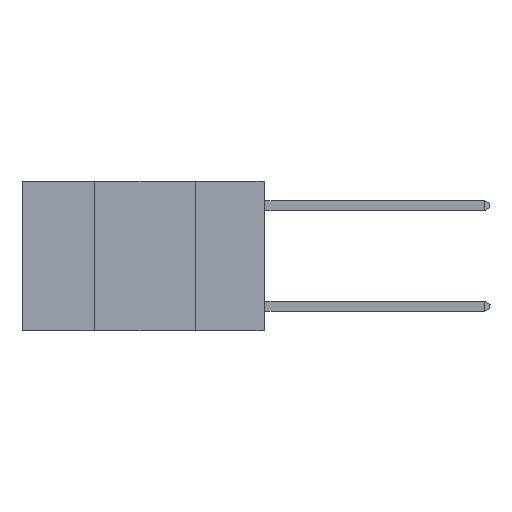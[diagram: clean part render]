
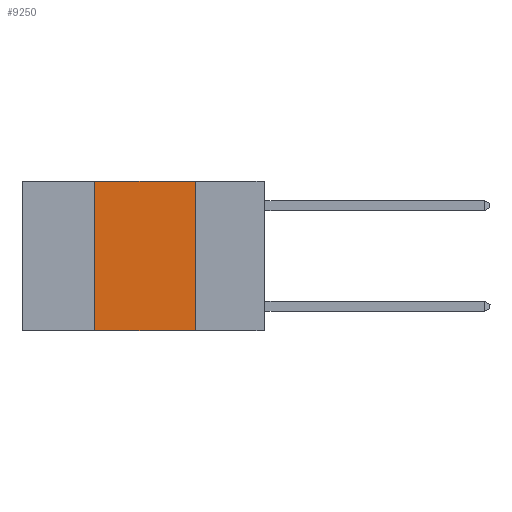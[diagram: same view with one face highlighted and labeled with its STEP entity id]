
A CAD part, left-side view. The second image highlights one B-rep face of the part: STEP entity #9250.
In plain terms, the highlighted planar face has unit normal (-1, 0, 0).
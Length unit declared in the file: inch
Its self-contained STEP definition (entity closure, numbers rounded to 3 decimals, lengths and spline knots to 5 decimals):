
#899 = VECTOR ( 'NONE', #6600, 39.37008 ) ;
#1778 = DIRECTION ( 'NONE',  ( 1., 0., 0. ) ) ;
#2074 = CARTESIAN_POINT ( 'NONE',  ( 0., 0.17, 0. ) ) ;
#2697 = DIRECTION ( 'NONE',  ( 0., -1., 0. ) ) ;
#2710 = VECTOR ( 'NONE', #13397, 39.37008 ) ;
#3205 = ORIENTED_EDGE ( 'NONE', *, *, #10799, .F. ) ;
#3374 = ORIENTED_EDGE ( 'NONE', *, *, #15927, .T. ) ;
#3683 = VERTEX_POINT ( 'NONE', #12729 ) ;
#3836 = LINE ( 'NONE', #6655, #899 ) ;
#3963 = EDGE_LOOP ( 'NONE', ( #3205, #9900, #13261, #3374 ) ) ;
#4249 = LINE ( 'NONE', #9937, #13894 ) ;
#5135 = CARTESIAN_POINT ( 'NONE',  ( 0., 0.17, -0.37 ) ) ;
#6184 = DIRECTION ( 'NONE',  ( 0., 0., 1. ) ) ;
#6420 = CARTESIAN_POINT ( 'NONE',  ( 0., 0.6, -0.37 ) ) ;
#6600 = DIRECTION ( 'NONE',  ( 0., -1., 0. ) ) ;
#6655 = CARTESIAN_POINT ( 'NONE',  ( 0., 0.6, 0. ) ) ;
#7323 = CARTESIAN_POINT ( 'NONE',  ( 0., 0.17, 0. ) ) ;
#8259 = EDGE_CURVE ( 'NONE', #11258, #3683, #4249, .T. ) ;
#8358 = VERTEX_POINT ( 'NONE', #5135 ) ;
#9023 = FACE_OUTER_BOUND ( 'NONE', #3963, .T. ) ;
#9250 = ADVANCED_FACE ( 'NONE', ( #9023 ), #9301, .F. ) ;
#9301 = PLANE ( 'NONE',  #9827 ) ;
#9405 = LINE ( 'NONE', #2074, #2710 ) ;
#9827 = AXIS2_PLACEMENT_3D ( 'NONE', #13056, #1778, #10556 ) ;
#9900 = ORIENTED_EDGE ( 'NONE', *, *, #12156, .F. ) ;
#9937 = CARTESIAN_POINT ( 'NONE',  ( 0., 0.42, 0. ) ) ;
#10055 = VECTOR ( 'NONE', #2697, 39.37008 ) ;
#10556 = DIRECTION ( 'NONE',  ( 0., 0., -1. ) ) ;
#10799 = EDGE_CURVE ( 'NONE', #11819, #8358, #9405, .T. ) ;
#11258 = VERTEX_POINT ( 'NONE', #16147 ) ;
#11819 = VERTEX_POINT ( 'NONE', #7323 ) ;
#12156 = EDGE_CURVE ( 'NONE', #3683, #11819, #3836, .T. ) ;
#12729 = CARTESIAN_POINT ( 'NONE',  ( 0., 0.42, 0. ) ) ;
#13056 = CARTESIAN_POINT ( 'NONE',  ( 0., 0.6, 0. ) ) ;
#13261 = ORIENTED_EDGE ( 'NONE', *, *, #8259, .F. ) ;
#13397 = DIRECTION ( 'NONE',  ( 0., 0., -1. ) ) ;
#13418 = LINE ( 'NONE', #6420, #10055 ) ;
#13894 = VECTOR ( 'NONE', #6184, 39.37008 ) ;
#15927 = EDGE_CURVE ( 'NONE', #11258, #8358, #13418, .T. ) ;
#16147 = CARTESIAN_POINT ( 'NONE',  ( 0., 0.42, -0.37 ) ) ;
